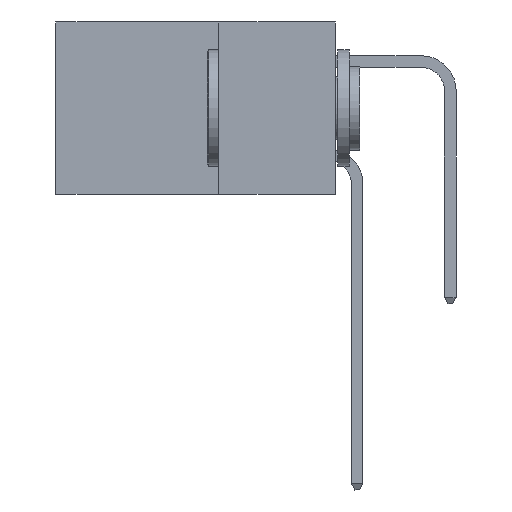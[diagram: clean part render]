
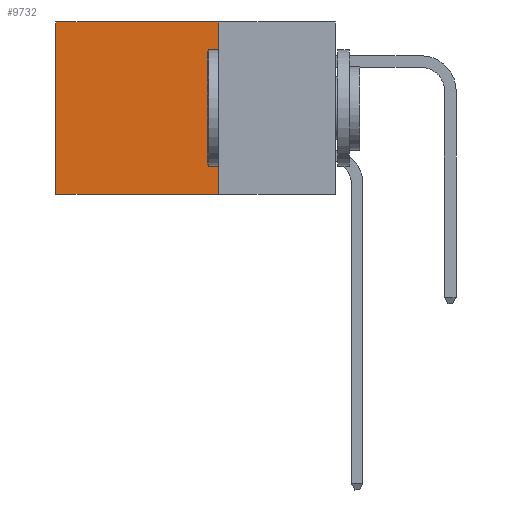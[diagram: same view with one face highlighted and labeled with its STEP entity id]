
A CAD part, left-side view. The second image highlights one B-rep face of the part: STEP entity #9732.
In plain terms, the highlighted planar face has unit normal (-1, 0, 0).
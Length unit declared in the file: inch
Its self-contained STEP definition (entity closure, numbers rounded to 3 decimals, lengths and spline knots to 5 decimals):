
#1394 = CARTESIAN_POINT ( 'NONE',  ( 0.2875, 0.25, 0. ) ) ;
#2783 = EDGE_LOOP ( 'NONE', ( #7896, #17931, #16483, #6073 ) ) ;
#4261 = LINE ( 'NONE', #14473, #5641 ) ;
#5623 = CARTESIAN_POINT ( 'NONE',  ( 0.2875, 0.25, 0. ) ) ;
#5641 = VECTOR ( 'NONE', #19760, 39.37008 ) ;
#6073 = ORIENTED_EDGE ( 'NONE', *, *, #22067, .T. ) ;
#6438 = VERTEX_POINT ( 'NONE', #7238 ) ;
#6517 = CARTESIAN_POINT ( 'NONE',  ( 0.2875, 0.6, 0. ) ) ;
#6600 = DIRECTION ( 'NONE',  ( 0., 0., -1. ) ) ;
#6605 = CARTESIAN_POINT ( 'NONE',  ( 0.2875, 0.6, -0.37 ) ) ;
#7129 = EDGE_CURVE ( 'NONE', #7557, #17688, #9190, .T. ) ;
#7238 = CARTESIAN_POINT ( 'NONE',  ( 0.2875, 0.25, -0.37 ) ) ;
#7557 = VERTEX_POINT ( 'NONE', #16695 ) ;
#7896 = ORIENTED_EDGE ( 'NONE', *, *, #7129, .T. ) ;
#9190 = LINE ( 'NONE', #6517, #15124 ) ;
#9732 = ADVANCED_FACE ( 'NONE', ( #19593 ), #13078, .F. ) ;
#10290 = DIRECTION ( 'NONE',  ( 0., 1., 0. ) ) ;
#10781 = VERTEX_POINT ( 'NONE', #5623 ) ;
#13078 = PLANE ( 'NONE',  #19180 ) ;
#14473 = CARTESIAN_POINT ( 'NONE',  ( 0.2875, 0.25, -0.37 ) ) ;
#14651 = DIRECTION ( 'NONE',  ( 0., 0., -1. ) ) ;
#14802 = CARTESIAN_POINT ( 'NONE',  ( 0.2875, 0.25, 0. ) ) ;
#15124 = VECTOR ( 'NONE', #6600, 39.37008 ) ;
#16483 = ORIENTED_EDGE ( 'NONE', *, *, #23118, .F. ) ;
#16651 = VECTOR ( 'NONE', #21964, 39.37008 ) ;
#16695 = CARTESIAN_POINT ( 'NONE',  ( 0.2875, 0.6, 0. ) ) ;
#16827 = EDGE_CURVE ( 'NONE', #6438, #17688, #4261, .T. ) ;
#17628 = VECTOR ( 'NONE', #10290, 39.37008 ) ;
#17688 = VERTEX_POINT ( 'NONE', #6605 ) ;
#17931 = ORIENTED_EDGE ( 'NONE', *, *, #16827, .F. ) ;
#19180 = AXIS2_PLACEMENT_3D ( 'NONE', #14802, #20408, #14651 ) ;
#19593 = FACE_OUTER_BOUND ( 'NONE', #2783, .T. ) ;
#19718 = CARTESIAN_POINT ( 'NONE',  ( 0.2875, 0.25, 0. ) ) ;
#19760 = DIRECTION ( 'NONE',  ( 0., 1., 0. ) ) ;
#19929 = LINE ( 'NONE', #1394, #17628 ) ;
#20408 = DIRECTION ( 'NONE',  ( 1., 0., 0. ) ) ;
#20677 = LINE ( 'NONE', #19718, #16651 ) ;
#21964 = DIRECTION ( 'NONE',  ( 0., 0., -1. ) ) ;
#22067 = EDGE_CURVE ( 'NONE', #10781, #7557, #19929, .T. ) ;
#23118 = EDGE_CURVE ( 'NONE', #10781, #6438, #20677, .T. ) ;
